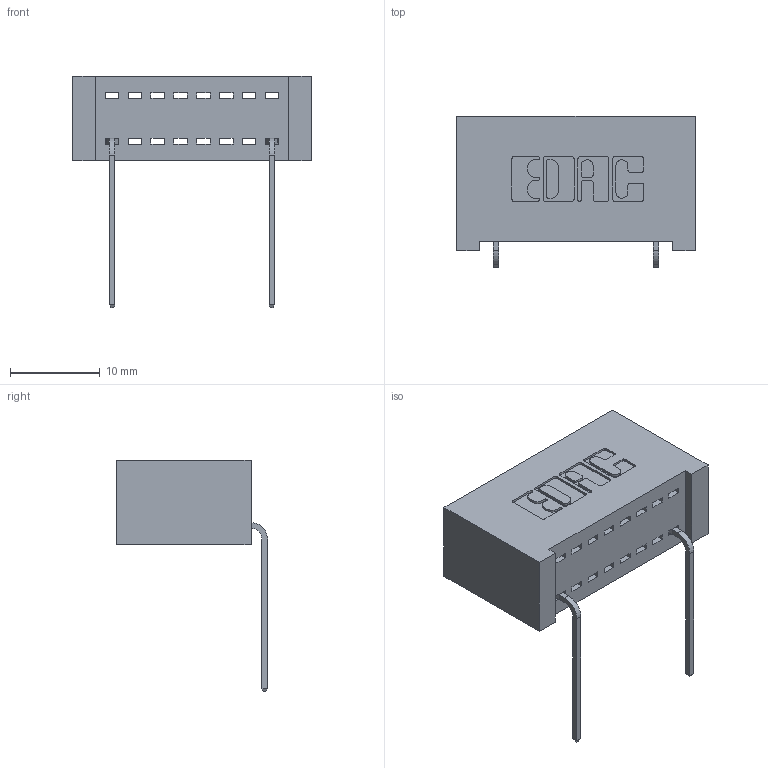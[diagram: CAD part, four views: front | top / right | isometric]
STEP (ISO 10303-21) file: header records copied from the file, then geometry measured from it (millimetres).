
FILE_DESCRIPTION (( 'STEP AP203' ), '1' );
FILE_NAME ('392-008-559-101.STEP', '2018-08-14T19:31:50', ( '' ), ( '' ), 'SwSTEP 2.0', 'SolidWorks 2016', '' );
FILE_SCHEMA (( 'CONFIG_CONTROL_DESIGN' ));
Length unit declared in the file: inch
Products named in the file (3): 342 Part_Lugless; 345-292-001_558 559 Tail - 1; 392-008-559-101
Assembly tree (3 placements, depth 2):
  392-008-559-101
    342 Part_Lugless
    345-292-001_558 559 Tail - 1  x2
Bounding box: 26.57 x 16.83 x 25.78 mm (x, y, z)
Volume: 2551.3 mm3; surface area: 3117.2 mm2
Topology: 3 solids, 3 shells, 294 faces, 891 edges, 590 vertices
Faces by surface type: plane 222, cylinder 72
Entity records: 8771 total; most frequent: CARTESIAN_POINT 1552, ORIENTED_EDGE 1502, DIRECTION 1363, EDGE_CURVE 751, VECTOR 631, LINE 631, VERTEX_POINT 498, AXIS2_PLACEMENT_3D 366
